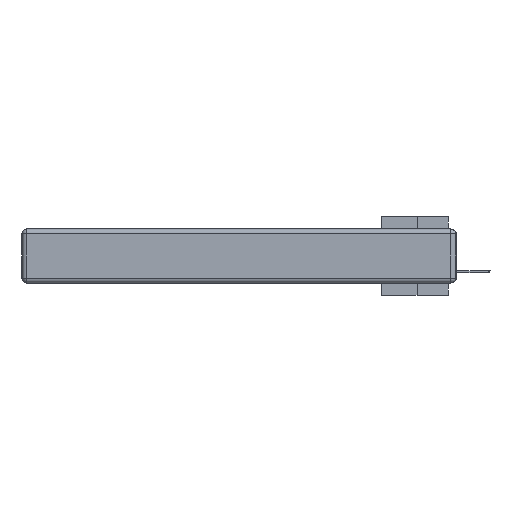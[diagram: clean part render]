
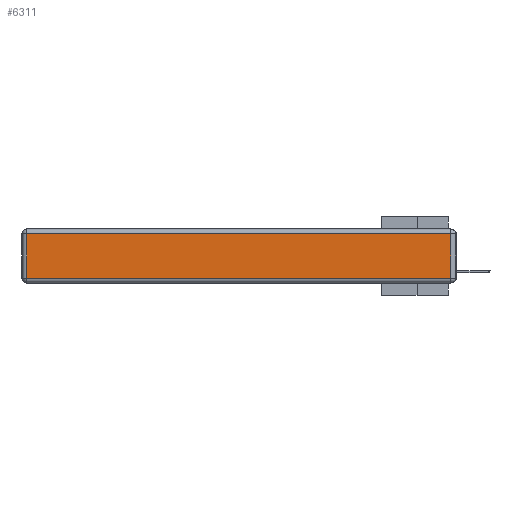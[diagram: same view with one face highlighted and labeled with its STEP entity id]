
A CAD part, left-side view. The second image highlights one B-rep face of the part: STEP entity #6311.
In plain terms, the highlighted planar face has unit normal (-1, 0, 0).
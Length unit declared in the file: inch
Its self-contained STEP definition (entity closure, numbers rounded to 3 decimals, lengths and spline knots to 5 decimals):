
#505 = DIRECTION ( 'NONE',  ( 0., 1., 0. ) ) ;
#795 = VERTEX_POINT ( 'NONE', #21851 ) ;
#1911 = CARTESIAN_POINT ( 'NONE',  ( 0., 2.72, -0.313 ) ) ;
#2802 = EDGE_CURVE ( 'NONE', #28759, #795, #13455, .T. ) ;
#3497 = EDGE_CURVE ( 'NONE', #795, #31423, #31345, .T. ) ;
#6311 = ADVANCED_FACE ( 'NONE', ( #18175 ), #33945, .T. ) ;
#6442 = AXIS2_PLACEMENT_3D ( 'NONE', #7762, #18346, #31863 ) ;
#7762 = CARTESIAN_POINT ( 'NONE',  ( 0., 0., -0.343 ) ) ;
#8573 = EDGE_LOOP ( 'NONE', ( #33772, #21561, #19246, #12474 ) ) ;
#10283 = CARTESIAN_POINT ( 'NONE',  ( 0., 2.72, -0.343 ) ) ;
#12474 = ORIENTED_EDGE ( 'NONE', *, *, #26354, .T. ) ;
#13455 = LINE ( 'NONE', #27295, #16453 ) ;
#16453 = VECTOR ( 'NONE', #32686, 39.37008 ) ;
#17884 = CARTESIAN_POINT ( 'NONE',  ( 0., 0.03, -0.03 ) ) ;
#18175 = FACE_OUTER_BOUND ( 'NONE', #8573, .T. ) ;
#18346 = DIRECTION ( 'NONE',  ( -1., 0., 0. ) ) ;
#19246 = ORIENTED_EDGE ( 'NONE', *, *, #30224, .T. ) ;
#21218 = LINE ( 'NONE', #24321, #30124 ) ;
#21561 = ORIENTED_EDGE ( 'NONE', *, *, #3497, .T. ) ;
#21851 = CARTESIAN_POINT ( 'NONE',  ( 0., 0.03, -0.313 ) ) ;
#22223 = VECTOR ( 'NONE', #23277, 39.37008 ) ;
#23277 = DIRECTION ( 'NONE',  ( 0., 0., -1. ) ) ;
#24321 = CARTESIAN_POINT ( 'NONE',  ( 0., 2.75, -0.03 ) ) ;
#24898 = VECTOR ( 'NONE', #31523, 39.37008 ) ;
#26225 = LINE ( 'NONE', #10283, #22223 ) ;
#26354 = EDGE_CURVE ( 'NONE', #27876, #28759, #26225, .T. ) ;
#27295 = CARTESIAN_POINT ( 'NONE',  ( 0., 0., -0.313 ) ) ;
#27876 = VERTEX_POINT ( 'NONE', #28548 ) ;
#28548 = CARTESIAN_POINT ( 'NONE',  ( 0., 2.72, -0.03 ) ) ;
#28759 = VERTEX_POINT ( 'NONE', #1911 ) ;
#30124 = VECTOR ( 'NONE', #505, 39.37008 ) ;
#30224 = EDGE_CURVE ( 'NONE', #31423, #27876, #21218, .T. ) ;
#31345 = LINE ( 'NONE', #33950, #24898 ) ;
#31423 = VERTEX_POINT ( 'NONE', #17884 ) ;
#31523 = DIRECTION ( 'NONE',  ( 0., 0., 1. ) ) ;
#31863 = DIRECTION ( 'NONE',  ( 0., 0., 1. ) ) ;
#32686 = DIRECTION ( 'NONE',  ( 0., -1., 0. ) ) ;
#33772 = ORIENTED_EDGE ( 'NONE', *, *, #2802, .T. ) ;
#33945 = PLANE ( 'NONE',  #6442 ) ;
#33950 = CARTESIAN_POINT ( 'NONE',  ( 0., 0.03, -0.343 ) ) ;
